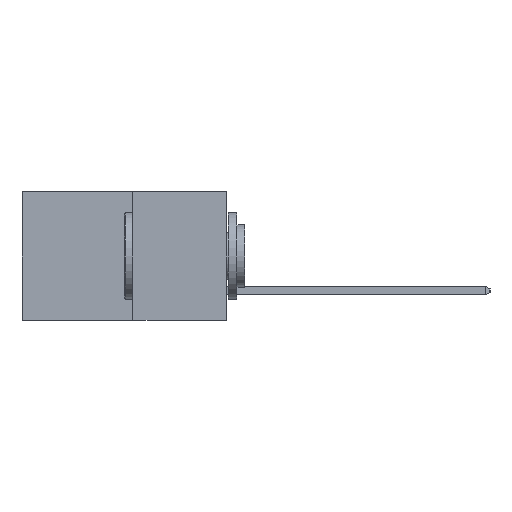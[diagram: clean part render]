
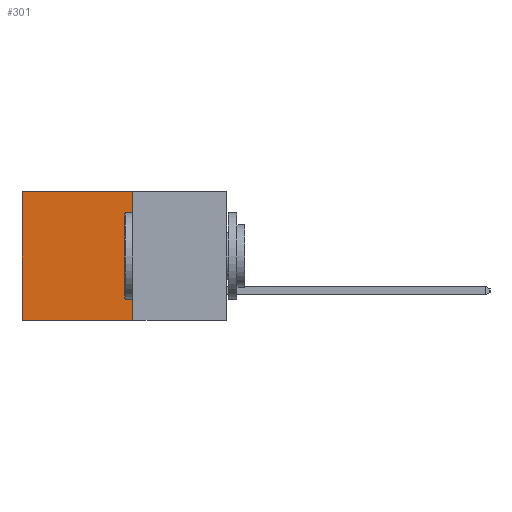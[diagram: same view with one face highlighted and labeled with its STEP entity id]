
A CAD part, left-side view. The second image highlights one B-rep face of the part: STEP entity #301.
In plain terms, the highlighted planar face has unit normal (-1, 0, 0).
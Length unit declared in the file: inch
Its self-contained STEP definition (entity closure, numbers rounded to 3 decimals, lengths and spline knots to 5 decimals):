
#270 = CARTESIAN_POINT ( 'NONE',  ( 0.277, 0.59, -0.37 ) ) ;
#301 = ADVANCED_FACE ( 'NONE', ( #10803 ), #2105, .F. ) ;
#884 = VERTEX_POINT ( 'NONE', #6522 ) ;
#1537 = EDGE_CURVE ( 'NONE', #4460, #5192, #5005, .T. ) ;
#1629 = VERTEX_POINT ( 'NONE', #9322 ) ;
#1974 = DIRECTION ( 'NONE',  ( 0., 0., -1. ) ) ;
#2105 = PLANE ( 'NONE',  #4329 ) ;
#2572 = EDGE_CURVE ( 'NONE', #4460, #884, #10770, .T. ) ;
#2827 = DIRECTION ( 'NONE',  ( 1., 0., 0. ) ) ;
#3172 = EDGE_CURVE ( 'NONE', #5192, #1629, #6946, .T. ) ;
#3431 = ORIENTED_EDGE ( 'NONE', *, *, #3172, .T. ) ;
#3508 = CARTESIAN_POINT ( 'NONE',  ( 0.277, 0.27, 0. ) ) ;
#3622 = LINE ( 'NONE', #8044, #8232 ) ;
#3708 = EDGE_CURVE ( 'NONE', #884, #1629, #3622, .T. ) ;
#3709 = ORIENTED_EDGE ( 'NONE', *, *, #2572, .F. ) ;
#4225 = VECTOR ( 'NONE', #1974, 39.37008 ) ;
#4294 = CARTESIAN_POINT ( 'NONE',  ( 0.277, 0.27, -0.37 ) ) ;
#4329 = AXIS2_PLACEMENT_3D ( 'NONE', #4294, #2827, #11339 ) ;
#4460 = VERTEX_POINT ( 'NONE', #8844 ) ;
#4743 = DIRECTION ( 'NONE',  ( 0., 1., 0. ) ) ;
#5005 = LINE ( 'NONE', #3508, #9545 ) ;
#5192 = VERTEX_POINT ( 'NONE', #11257 ) ;
#6522 = CARTESIAN_POINT ( 'NONE',  ( 0.277, 0.27, -0.37 ) ) ;
#6610 = CARTESIAN_POINT ( 'NONE',  ( 0.277, 0.27, -0.37 ) ) ;
#6946 = LINE ( 'NONE', #270, #4225 ) ;
#7858 = DIRECTION ( 'NONE',  ( 0., 1., 0. ) ) ;
#8044 = CARTESIAN_POINT ( 'NONE',  ( 0.277, 0.27, -0.37 ) ) ;
#8232 = VECTOR ( 'NONE', #7858, 39.37008 ) ;
#8321 = ORIENTED_EDGE ( 'NONE', *, *, #3708, .F. ) ;
#8599 = ORIENTED_EDGE ( 'NONE', *, *, #1537, .T. ) ;
#8844 = CARTESIAN_POINT ( 'NONE',  ( 0.277, 0.27, 0. ) ) ;
#9322 = CARTESIAN_POINT ( 'NONE',  ( 0.277, 0.59, -0.37 ) ) ;
#9545 = VECTOR ( 'NONE', #4743, 39.37008 ) ;
#10215 = DIRECTION ( 'NONE',  ( 0., 0., -1. ) ) ;
#10770 = LINE ( 'NONE', #6610, #11038 ) ;
#10803 = FACE_OUTER_BOUND ( 'NONE', #11624, .T. ) ;
#11038 = VECTOR ( 'NONE', #10215, 39.37008 ) ;
#11257 = CARTESIAN_POINT ( 'NONE',  ( 0.277, 0.59, 0. ) ) ;
#11339 = DIRECTION ( 'NONE',  ( 0., 0., -1. ) ) ;
#11624 = EDGE_LOOP ( 'NONE', ( #3431, #8321, #3709, #8599 ) ) ;
